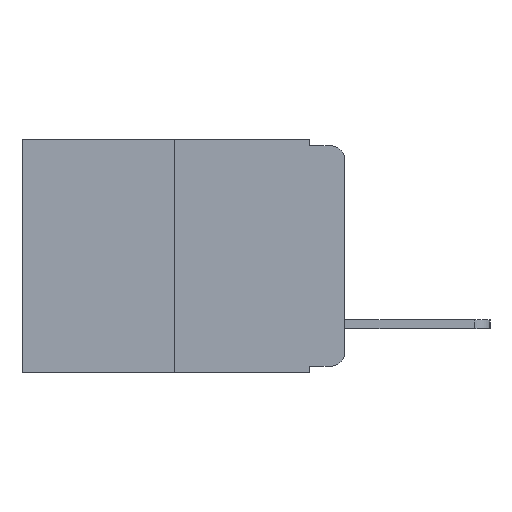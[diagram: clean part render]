
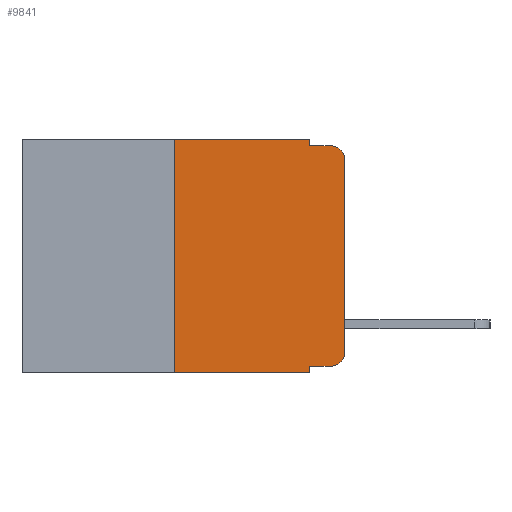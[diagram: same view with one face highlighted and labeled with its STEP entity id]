
A CAD part, left-side view. The second image highlights one B-rep face of the part: STEP entity #9841.
In plain terms, the highlighted planar face has unit normal (-1, 0, 0).
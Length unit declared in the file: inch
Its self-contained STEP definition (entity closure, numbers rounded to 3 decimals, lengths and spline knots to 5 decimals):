
#155 = CARTESIAN_POINT ( 'NONE',  ( 0., 0.051, -0.333 ) ) ;
#294 = PLANE ( 'NONE',  #4198 ) ;
#441 = DIRECTION ( 'NONE',  ( -1., 0., 0. ) ) ;
#474 = ORIENTED_EDGE ( 'NONE', *, *, #4081, .F. ) ;
#641 = CARTESIAN_POINT ( 'NONE',  ( 0., 0.02, -0.01 ) ) ;
#685 = VERTEX_POINT ( 'NONE', #6514 ) ;
#890 = VERTEX_POINT ( 'NONE', #641 ) ;
#937 = CARTESIAN_POINT ( 'NONE',  ( 0., 0.25, 0. ) ) ;
#988 = ORIENTED_EDGE ( 'NONE', *, *, #9566, .T. ) ;
#1294 = VERTEX_POINT ( 'NONE', #8998 ) ;
#1548 = CARTESIAN_POINT ( 'NONE',  ( 0., 0.473, 0. ) ) ;
#1553 = CARTESIAN_POINT ( 'NONE',  ( 0., 0.02, -0.333 ) ) ;
#1695 = LINE ( 'NONE', #7942, #8519 ) ;
#1731 = FACE_OUTER_BOUND ( 'NONE', #3137, .T. ) ;
#2251 = VERTEX_POINT ( 'NONE', #155 ) ;
#2330 = ORIENTED_EDGE ( 'NONE', *, *, #4125, .F. ) ;
#2621 = CARTESIAN_POINT ( 'NONE',  ( 0., 0.25, 0. ) ) ;
#2864 = CIRCLE ( 'NONE', #8276, 0.02 ) ;
#2875 = VECTOR ( 'NONE', #4931, 39.37008 ) ;
#3082 = VECTOR ( 'NONE', #10366, 39.37008 ) ;
#3137 = EDGE_LOOP ( 'NONE', ( #4972, #9144, #9447, #9999, #10869, #474, #988, #2330, #5514, #7711 ) ) ;
#3207 = AXIS2_PLACEMENT_3D ( 'NONE', #9324, #10003, #9705 ) ;
#3262 = DIRECTION ( 'NONE',  ( 0., 0., -1. ) ) ;
#3500 = CARTESIAN_POINT ( 'NONE',  ( 0., 0., -0.03 ) ) ;
#3847 = EDGE_CURVE ( 'NONE', #7870, #4566, #5060, .T. ) ;
#3860 = EDGE_CURVE ( 'NONE', #4566, #890, #7172, .T. ) ;
#3896 = EDGE_CURVE ( 'NONE', #685, #890, #4496, .T. ) ;
#3979 = EDGE_CURVE ( 'NONE', #1294, #685, #1695, .T. ) ;
#4081 = EDGE_CURVE ( 'NONE', #5463, #7485, #6054, .T. ) ;
#4114 = VERTEX_POINT ( 'NONE', #1553 ) ;
#4125 = EDGE_CURVE ( 'NONE', #2251, #8314, #4905, .T. ) ;
#4149 = EDGE_CURVE ( 'NONE', #2251, #4114, #11164, .T. ) ;
#4198 = AXIS2_PLACEMENT_3D ( 'NONE', #10782, #8483, #3262 ) ;
#4239 = CARTESIAN_POINT ( 'NONE',  ( 0., 0., -0.313 ) ) ;
#4422 = EDGE_CURVE ( 'NONE', #4114, #7870, #2864, .T. ) ;
#4496 = LINE ( 'NONE', #4944, #2875 ) ;
#4557 = CARTESIAN_POINT ( 'NONE',  ( 0., 0.473, -0.343 ) ) ;
#4566 = VERTEX_POINT ( 'NONE', #3500 ) ;
#4827 = DIRECTION ( 'NONE',  ( 0., 0., -1. ) ) ;
#4905 = LINE ( 'NONE', #6746, #9132 ) ;
#4931 = DIRECTION ( 'NONE',  ( 0., -1., 0. ) ) ;
#4944 = CARTESIAN_POINT ( 'NONE',  ( 0., 0.051, -0.01 ) ) ;
#4972 = ORIENTED_EDGE ( 'NONE', *, *, #3847, .T. ) ;
#5060 = LINE ( 'NONE', #8802, #5628 ) ;
#5463 = VERTEX_POINT ( 'NONE', #8871 ) ;
#5487 = VECTOR ( 'NONE', #8118, 39.37008 ) ;
#5514 = ORIENTED_EDGE ( 'NONE', *, *, #4149, .T. ) ;
#5628 = VECTOR ( 'NONE', #11242, 39.37008 ) ;
#5857 = DIRECTION ( 'NONE',  ( 0., -1., 0. ) ) ;
#6054 = LINE ( 'NONE', #2621, #5487 ) ;
#6514 = CARTESIAN_POINT ( 'NONE',  ( 0., 0.051, -0.01 ) ) ;
#6746 = CARTESIAN_POINT ( 'NONE',  ( 0., 0.051, 0. ) ) ;
#7172 = CIRCLE ( 'NONE', #3207, 0.02 ) ;
#7485 = VERTEX_POINT ( 'NONE', #937 ) ;
#7711 = ORIENTED_EDGE ( 'NONE', *, *, #4422, .T. ) ;
#7870 = VERTEX_POINT ( 'NONE', #4239 ) ;
#7942 = CARTESIAN_POINT ( 'NONE',  ( 0., 0.051, 0. ) ) ;
#8118 = DIRECTION ( 'NONE',  ( 0., 0., 1. ) ) ;
#8146 = VECTOR ( 'NONE', #10987, 39.37008 ) ;
#8225 = CARTESIAN_POINT ( 'NONE',  ( 0., 0.051, -0.343 ) ) ;
#8276 = AXIS2_PLACEMENT_3D ( 'NONE', #10069, #441, #9601 ) ;
#8314 = VERTEX_POINT ( 'NONE', #8225 ) ;
#8483 = DIRECTION ( 'NONE',  ( 1., 0., 0. ) ) ;
#8519 = VECTOR ( 'NONE', #10721, 39.37008 ) ;
#8802 = CARTESIAN_POINT ( 'NONE',  ( 0., 0., 0. ) ) ;
#8871 = CARTESIAN_POINT ( 'NONE',  ( 0., 0.25, -0.343 ) ) ;
#8888 = VECTOR ( 'NONE', #5857, 39.37008 ) ;
#8998 = CARTESIAN_POINT ( 'NONE',  ( 0., 0.051, 0. ) ) ;
#9003 = CARTESIAN_POINT ( 'NONE',  ( 0., 0.051, -0.333 ) ) ;
#9132 = VECTOR ( 'NONE', #4827, 39.37008 ) ;
#9144 = ORIENTED_EDGE ( 'NONE', *, *, #3860, .T. ) ;
#9324 = CARTESIAN_POINT ( 'NONE',  ( 0., 0.02, -0.03 ) ) ;
#9447 = ORIENTED_EDGE ( 'NONE', *, *, #3896, .F. ) ;
#9566 = EDGE_CURVE ( 'NONE', #5463, #8314, #9675, .T. ) ;
#9601 = DIRECTION ( 'NONE',  ( 0., 0., -1. ) ) ;
#9675 = LINE ( 'NONE', #4557, #3082 ) ;
#9705 = DIRECTION ( 'NONE',  ( 0., 0., -1. ) ) ;
#9841 = ADVANCED_FACE ( 'NONE', ( #1731 ), #294, .F. ) ;
#9999 = ORIENTED_EDGE ( 'NONE', *, *, #3979, .F. ) ;
#10003 = DIRECTION ( 'NONE',  ( -1., 0., 0. ) ) ;
#10069 = CARTESIAN_POINT ( 'NONE',  ( 0., 0.02, -0.313 ) ) ;
#10366 = DIRECTION ( 'NONE',  ( 0., -1., 0. ) ) ;
#10471 = LINE ( 'NONE', #1548, #8146 ) ;
#10721 = DIRECTION ( 'NONE',  ( 0., 0., -1. ) ) ;
#10747 = EDGE_CURVE ( 'NONE', #7485, #1294, #10471, .T. ) ;
#10782 = CARTESIAN_POINT ( 'NONE',  ( 0., 0.473, 0. ) ) ;
#10869 = ORIENTED_EDGE ( 'NONE', *, *, #10747, .F. ) ;
#10987 = DIRECTION ( 'NONE',  ( 0., -1., 0. ) ) ;
#11164 = LINE ( 'NONE', #9003, #8888 ) ;
#11242 = DIRECTION ( 'NONE',  ( 0., 0., 1. ) ) ;
